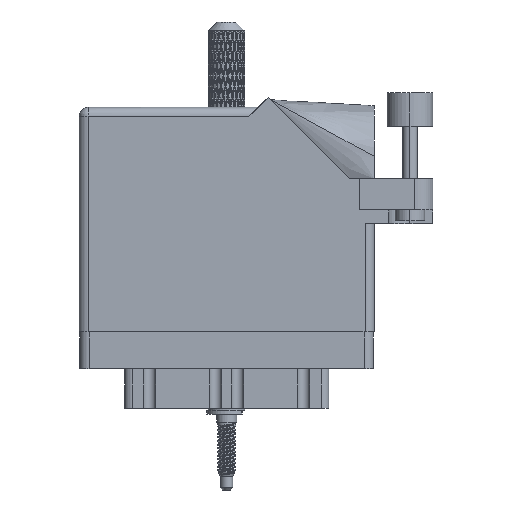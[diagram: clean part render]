
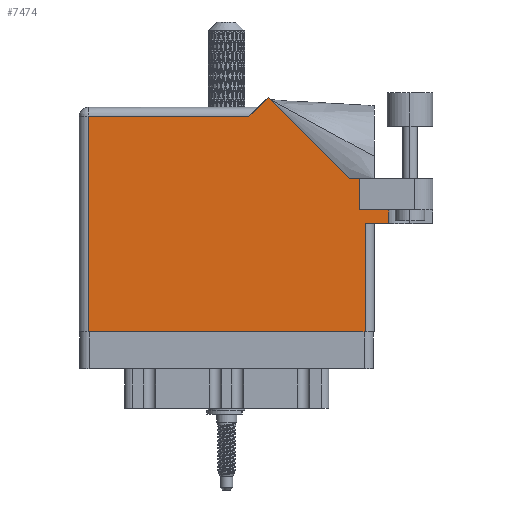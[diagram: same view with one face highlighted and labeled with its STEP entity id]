
A CAD part, front view. The second image highlights one B-rep face of the part: STEP entity #7474.
In plain terms, the highlighted face is planar.
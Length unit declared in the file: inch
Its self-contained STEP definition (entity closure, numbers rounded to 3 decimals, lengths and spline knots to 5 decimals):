
#916 = ORIENTED_EDGE ( 'NONE', *, *, #40294, .T. ) ;
#1031 = DIRECTION ( 'NONE',  ( 0., 1., 0. ) ) ;
#1032 = EDGE_CURVE ( 'NONE', #78748, #79436, #14094, .T. ) ;
#1233 = LINE ( 'NONE', #76099, #91656 ) ;
#2704 = VERTEX_POINT ( 'NONE', #28806 ) ;
#3132 = CARTESIAN_POINT ( 'NONE',  ( 1.84442, 1.044, 0. ) ) ;
#7474 = ADVANCED_FACE ( 'NONE', ( #66926 ), #65875, .F. ) ;
#7988 = DIRECTION ( 'NONE',  ( 0., 0., -1. ) ) ;
#10358 = ORIENTED_EDGE ( 'NONE', *, *, #50487, .T. ) ;
#11657 = VERTEX_POINT ( 'NONE', #44744 ) ;
#11775 = VECTOR ( 'NONE', #71273, 39.37008 ) ;
#13369 = VECTOR ( 'NONE', #56567, 39.37008 ) ;
#14094 = LINE ( 'NONE', #61390, #44991 ) ;
#14685 = CARTESIAN_POINT ( 'NONE',  ( 2.1115, 0.831, 0. ) ) ;
#14722 = VECTOR ( 'NONE', #25366, 39.37008 ) ;
#16626 = ORIENTED_EDGE ( 'NONE', *, *, #53128, .F. ) ;
#18367 = VECTOR ( 'NONE', #34229, 39.37008 ) ;
#20465 = ORIENTED_EDGE ( 'NONE', *, *, #103759, .T. ) ;
#20648 = EDGE_CURVE ( 'NONE', #80844, #78748, #50854, .T. ) ;
#24779 = CARTESIAN_POINT ( 'NONE',  ( 0., 0., 0. ) ) ;
#24836 = DIRECTION ( 'NONE',  ( 1., 0., 0. ) ) ;
#25366 = DIRECTION ( 'NONE',  ( -0.707, -0.707, 0. ) ) ;
#26156 = VECTOR ( 'NONE', #51975, 39.37008 ) ;
#26519 = CARTESIAN_POINT ( 'NONE',  ( 0., 1.53, 0. ) ) ;
#27221 = DIRECTION ( 'NONE',  ( 0., -1., 0. ) ) ;
#28806 = CARTESIAN_POINT ( 'NONE',  ( 1.91, 0.831, 0. ) ) ;
#29517 = EDGE_CURVE ( 'NONE', #11657, #31665, #104950, .T. ) ;
#31134 = CARTESIAN_POINT ( 'NONE',  ( 1.948, 0.737, 0. ) ) ;
#31665 = VERTEX_POINT ( 'NONE', #100325 ) ;
#31816 = LINE ( 'NONE', #97174, #39265 ) ;
#34229 = DIRECTION ( 'NONE',  ( 1., 0., 0. ) ) ;
#37794 = VERTEX_POINT ( 'NONE', #102786 ) ;
#38589 = EDGE_CURVE ( 'NONE', #2704, #74619, #43264, .T. ) ;
#39265 = VECTOR ( 'NONE', #1031, 39.37008 ) ;
#40294 = EDGE_CURVE ( 'NONE', #61630, #85853, #70243, .T. ) ;
#42674 = CARTESIAN_POINT ( 'NONE',  ( 0.062, 0., 0. ) ) ;
#43264 = LINE ( 'NONE', #99041, #18367 ) ;
#44026 = CARTESIAN_POINT ( 'NONE',  ( 1.84442, 1.044, 0. ) ) ;
#44744 = CARTESIAN_POINT ( 'NONE',  ( 1.948, 0., 0. ) ) ;
#44991 = VECTOR ( 'NONE', #62411, 39.37008 ) ;
#46690 = VERTEX_POINT ( 'NONE', #42674 ) ;
#46884 = AXIS2_PLACEMENT_3D ( 'NONE', #26519, #7988, #73334 ) ;
#48489 = CARTESIAN_POINT ( 'NONE',  ( 1.28771, 1.60071, 0. ) ) ;
#49806 = CARTESIAN_POINT ( 'NONE',  ( 1.217, 1.53, 0. ) ) ;
#49887 = EDGE_CURVE ( 'NONE', #46690, #11657, #97563, .T. ) ;
#50487 = EDGE_CURVE ( 'NONE', #85853, #80844, #75884, .T. ) ;
#50854 = LINE ( 'NONE', #49806, #14722 ) ;
#51975 = DIRECTION ( 'NONE',  ( -0.707, 0.707, 0. ) ) ;
#53128 = EDGE_CURVE ( 'NONE', #74619, #37794, #87383, .T. ) ;
#53741 = CARTESIAN_POINT ( 'NONE',  ( 2.41, 1.044, 0. ) ) ;
#56567 = DIRECTION ( 'NONE',  ( 0., -1., 0. ) ) ;
#61390 = CARTESIAN_POINT ( 'NONE',  ( 0., 1.468, 0. ) ) ;
#61630 = VERTEX_POINT ( 'NONE', #94068 ) ;
#62411 = DIRECTION ( 'NONE',  ( -1., 0., 0. ) ) ;
#62902 = ORIENTED_EDGE ( 'NONE', *, *, #78071, .T. ) ;
#63398 = VECTOR ( 'NONE', #83054, 39.37008 ) ;
#63784 = ORIENTED_EDGE ( 'NONE', *, *, #20648, .T. ) ;
#65139 = DIRECTION ( 'NONE',  ( 0., 1., 0. ) ) ;
#65728 = LINE ( 'NONE', #73185, #96751 ) ;
#65875 = PLANE ( 'NONE',  #46884 ) ;
#66926 = FACE_OUTER_BOUND ( 'NONE', #73508, .T. ) ;
#68792 = ORIENTED_EDGE ( 'NONE', *, *, #38589, .F. ) ;
#70243 = LINE ( 'NONE', #53741, #11775 ) ;
#71273 = DIRECTION ( 'NONE',  ( -1., 0., 0. ) ) ;
#72287 = CARTESIAN_POINT ( 'NONE',  ( 0.062, 1.468, 0. ) ) ;
#73185 = CARTESIAN_POINT ( 'NONE',  ( 2.01, 0.737, 0. ) ) ;
#73334 = DIRECTION ( 'NONE',  ( -1., 0., 0. ) ) ;
#73508 = EDGE_LOOP ( 'NONE', ( #74617, #82724, #62902, #16626, #68792, #20465, #916, #10358, #63784, #84675, #74652 ) ) ;
#74617 = ORIENTED_EDGE ( 'NONE', *, *, #49887, .T. ) ;
#74619 = VERTEX_POINT ( 'NONE', #14685 ) ;
#74652 = ORIENTED_EDGE ( 'NONE', *, *, #82049, .T. ) ;
#75884 = LINE ( 'NONE', #3132, #26156 ) ;
#76099 = CARTESIAN_POINT ( 'NONE',  ( 0.062, 0., 0. ) ) ;
#78071 = EDGE_CURVE ( 'NONE', #31665, #37794, #65728, .T. ) ;
#78748 = VERTEX_POINT ( 'NONE', #85871 ) ;
#79436 = VERTEX_POINT ( 'NONE', #72287 ) ;
#80844 = VERTEX_POINT ( 'NONE', #48489 ) ;
#82049 = EDGE_CURVE ( 'NONE', #79436, #46690, #1233, .T. ) ;
#82724 = ORIENTED_EDGE ( 'NONE', *, *, #29517, .T. ) ;
#83054 = DIRECTION ( 'NONE',  ( 1., 0., 0. ) ) ;
#84675 = ORIENTED_EDGE ( 'NONE', *, *, #1032, .T. ) ;
#85853 = VERTEX_POINT ( 'NONE', #44026 ) ;
#85871 = CARTESIAN_POINT ( 'NONE',  ( 1.155, 1.468, 0. ) ) ;
#87383 = LINE ( 'NONE', #96393, #13369 ) ;
#91656 = VECTOR ( 'NONE', #27221, 39.37008 ) ;
#93549 = VECTOR ( 'NONE', #65139, 39.37008 ) ;
#94068 = CARTESIAN_POINT ( 'NONE',  ( 1.91, 1.044, 0. ) ) ;
#96393 = CARTESIAN_POINT ( 'NONE',  ( 2.1115, 1.16177, 0. ) ) ;
#96751 = VECTOR ( 'NONE', #24836, 39.37008 ) ;
#97174 = CARTESIAN_POINT ( 'NONE',  ( 1.91, 0.831, 0. ) ) ;
#97563 = LINE ( 'NONE', #24779, #63398 ) ;
#99041 = CARTESIAN_POINT ( 'NONE',  ( 1.91, 0.831, 0. ) ) ;
#100325 = CARTESIAN_POINT ( 'NONE',  ( 1.948, 0.737, 0. ) ) ;
#102786 = CARTESIAN_POINT ( 'NONE',  ( 2.1115, 0.737, 0. ) ) ;
#103759 = EDGE_CURVE ( 'NONE', #2704, #61630, #31816, .T. ) ;
#104950 = LINE ( 'NONE', #31134, #93549 ) ;
